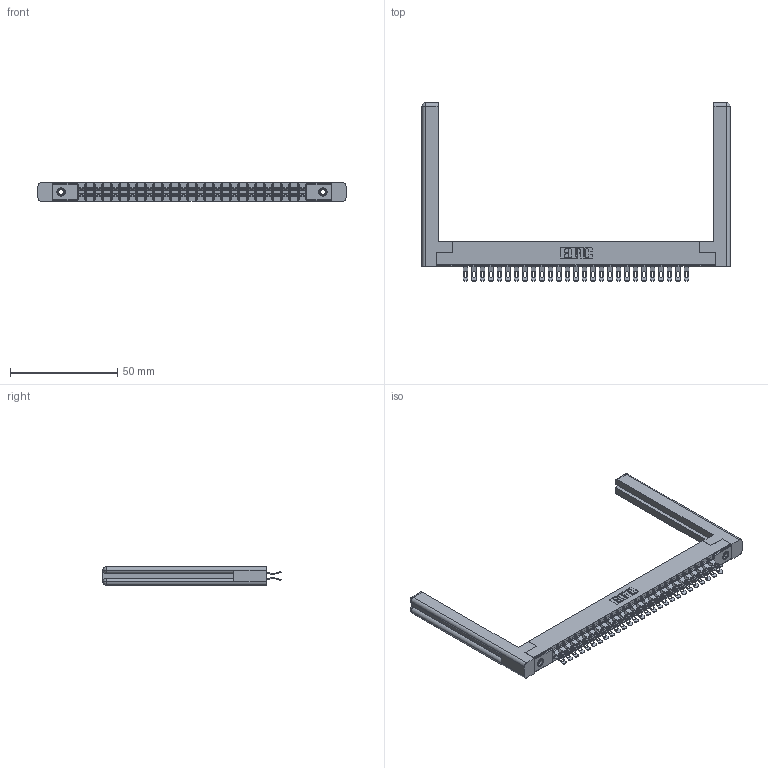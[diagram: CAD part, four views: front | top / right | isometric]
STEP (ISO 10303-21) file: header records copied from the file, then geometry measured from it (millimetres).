
FILE_DESCRIPTION (( 'STEP AP203' ), '1' );
FILE_NAME ('305-054-555-558.STEP', '2019-09-09T23:15:18', ( '' ), ( '' ), 'SwSTEP 2.0', 'SolidWorks 2016', '' );
FILE_SCHEMA (( 'CONFIG_CONTROL_DESIGN' ));
Length unit declared in the file: inch
Products named in the file (5): 307-220-058; 305-290-001_555; 305-054-555-558; 305 Part_.156 Dia; 345-250-001_345-250-001-102
Assembly tree (59 placements, depth 2):
  305-054-555-558
    305 Part_.156 Dia
    305-290-001_555  x54
    345-250-001_345-250-001-102  x2
    307-220-058  x2
Bounding box: 143.61 x 83.06 x 8.71 mm (x, y, z)
Volume: 16506.9 mm3; surface area: 23681.1 mm2
Topology: 59 solids, 59 shells, 3822 faces, 11335 edges, 7398 vertices
Faces by surface type: plane 1880, cylinder 1810, sphere 108, cone 12, torus 12
Entity records: 34317 total; most frequent: CARTESIAN_POINT 5712, ORIENTED_EDGE 5600, DIRECTION 5494, EDGE_CURVE 2800, LINE 2218, VECTOR 2218, VERTEX_POINT 1786, AXIS2_PLACEMENT_3D 1638
